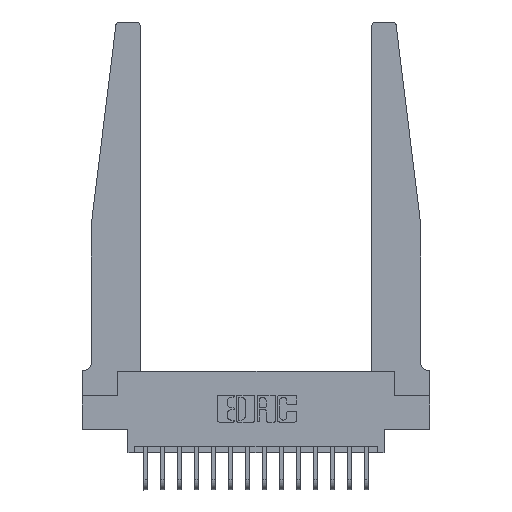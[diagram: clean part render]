
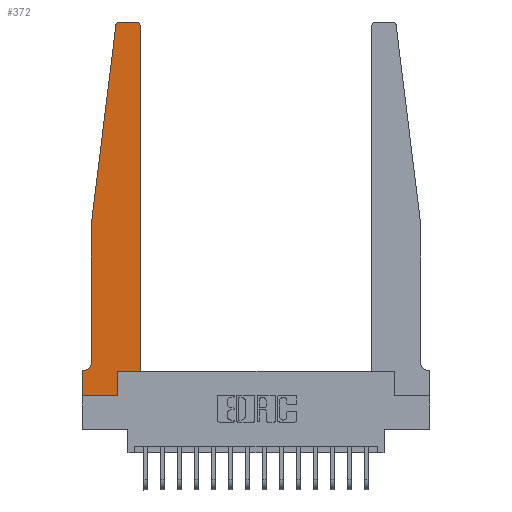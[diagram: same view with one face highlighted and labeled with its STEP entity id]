
A CAD part, top view. The second image highlights one B-rep face of the part: STEP entity #372.
In plain terms, the highlighted planar face has unit normal (0, 0, 1).
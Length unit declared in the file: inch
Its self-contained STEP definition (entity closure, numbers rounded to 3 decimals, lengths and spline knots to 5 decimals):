
#316 = CARTESIAN_POINT ( 'NONE',  ( 0.425, 2.72, 0.37 ) ) ;
#372 = ADVANCED_FACE ( 'NONE', ( #7397 ), #8404, .T. ) ;
#422 = DIRECTION ( 'NONE',  ( 0., -1., 0. ) ) ;
#849 = EDGE_CURVE ( 'NONE', #1952, #6375, #15134, .T. ) ;
#1084 = VERTEX_POINT ( 'NONE', #10043 ) ;
#1203 = DIRECTION ( 'NONE',  ( 1., 0., 0. ) ) ;
#1388 = ORIENTED_EDGE ( 'NONE', *, *, #10476, .T. ) ;
#1481 = DIRECTION ( 'NONE',  ( 1., 0., 0. ) ) ;
#1496 = CARTESIAN_POINT ( 'NONE',  ( 0.065, 1.25, 0.37 ) ) ;
#1817 = LINE ( 'NONE', #8762, #2252 ) ;
#1832 = ORIENTED_EDGE ( 'NONE', *, *, #15131, .T. ) ;
#1952 = VERTEX_POINT ( 'NONE', #4308 ) ;
#2252 = VECTOR ( 'NONE', #422, 39.37008 ) ;
#2431 = VERTEX_POINT ( 'NONE', #12686 ) ;
#2647 = DIRECTION ( 'NONE',  ( 0., 0., 1. ) ) ;
#3090 = EDGE_CURVE ( 'NONE', #2431, #8237, #17460, .T. ) ;
#3104 = CIRCLE ( 'NONE', #5356, 0.03 ) ;
#3363 = CARTESIAN_POINT ( 'NONE',  ( 0.2605, 0., 0.37 ) ) ;
#3645 = VECTOR ( 'NONE', #12883, 39.37008 ) ;
#3650 = DIRECTION ( 'NONE',  ( 0., -1., 0. ) ) ;
#3750 = LINE ( 'NONE', #11215, #17449 ) ;
#3850 = EDGE_CURVE ( 'NONE', #4819, #7649, #10717, .T. ) ;
#3952 = VECTOR ( 'NONE', #7969, 39.37008 ) ;
#3996 = VECTOR ( 'NONE', #4286, 39.37008 ) ;
#4286 = DIRECTION ( 'NONE',  ( -1., 0., 0. ) ) ;
#4308 = CARTESIAN_POINT ( 'NONE',  ( 0.2605, 0.18, 0.37 ) ) ;
#4644 = EDGE_LOOP ( 'NONE', ( #8132, #11613, #5805, #14864, #8345, #15280, #1388, #15687, #1832, #5587, #13024, #16502 ) ) ;
#4819 = VERTEX_POINT ( 'NONE', #11086 ) ;
#5010 = CARTESIAN_POINT ( 'NONE',  ( 0., 0., 0.37 ) ) ;
#5356 = AXIS2_PLACEMENT_3D ( 'NONE', #5907, #15098, #7273 ) ;
#5502 = DIRECTION ( 'NONE',  ( 0., 0., -1. ) ) ;
#5587 = ORIENTED_EDGE ( 'NONE', *, *, #849, .T. ) ;
#5805 = ORIENTED_EDGE ( 'NONE', *, *, #6548, .T. ) ;
#5907 = CARTESIAN_POINT ( 'NONE',  ( 0.395, 2.72, 0.37 ) ) ;
#6087 = EDGE_CURVE ( 'NONE', #7649, #11909, #7371, .T. ) ;
#6375 = VERTEX_POINT ( 'NONE', #15170 ) ;
#6548 = EDGE_CURVE ( 'NONE', #11909, #10144, #7354, .T. ) ;
#6642 = CARTESIAN_POINT ( 'NONE',  ( 0.25, 2.75, 0.37 ) ) ;
#7003 = VERTEX_POINT ( 'NONE', #316 ) ;
#7191 = AXIS2_PLACEMENT_3D ( 'NONE', #13401, #5502, #14726 ) ;
#7273 = DIRECTION ( 'NONE',  ( 1., 0., 0. ) ) ;
#7354 = LINE ( 'NONE', #16759, #3645 ) ;
#7371 = CIRCLE ( 'NONE', #9547, 0.03 ) ;
#7397 = FACE_OUTER_BOUND ( 'NONE', #4644, .T. ) ;
#7649 = VERTEX_POINT ( 'NONE', #15249 ) ;
#7888 = CIRCLE ( 'NONE', #7191, 0.05 ) ;
#7969 = DIRECTION ( 'NONE',  ( -1., 0., 0. ) ) ;
#8132 = ORIENTED_EDGE ( 'NONE', *, *, #3850, .T. ) ;
#8186 = CARTESIAN_POINT ( 'NONE',  ( 0., 0.1875, 0.37 ) ) ;
#8237 = VERTEX_POINT ( 'NONE', #3363 ) ;
#8341 = CARTESIAN_POINT ( 'NONE',  ( 0., 0.1875, 0.37 ) ) ;
#8345 = ORIENTED_EDGE ( 'NONE', *, *, #13932, .T. ) ;
#8404 = PLANE ( 'NONE',  #12423 ) ;
#8734 = EDGE_CURVE ( 'NONE', #10144, #1084, #1817, .T. ) ;
#8762 = CARTESIAN_POINT ( 'NONE',  ( 0.065, 1.25, 0.37 ) ) ;
#9404 = CARTESIAN_POINT ( 'NONE',  ( 0.015, 0.1875, 0.37 ) ) ;
#9446 = VECTOR ( 'NONE', #1203, 39.37008 ) ;
#9547 = AXIS2_PLACEMENT_3D ( 'NONE', #10792, #2647, #12108 ) ;
#9602 = EDGE_CURVE ( 'NONE', #16678, #16761, #14619, .T. ) ;
#9721 = DIRECTION ( 'NONE',  ( 0., 0., 1. ) ) ;
#9798 = CARTESIAN_POINT ( 'NONE',  ( 0.2605, 0.18, 0.37 ) ) ;
#10043 = CARTESIAN_POINT ( 'NONE',  ( 0.065, 0.2375, 0.37 ) ) ;
#10144 = VERTEX_POINT ( 'NONE', #1496 ) ;
#10476 = EDGE_CURVE ( 'NONE', #16761, #2431, #12675, .T. ) ;
#10717 = LINE ( 'NONE', #6642, #3952 ) ;
#10778 = CARTESIAN_POINT ( 'NONE',  ( 0.425, 0.18, 0.37 ) ) ;
#10792 = CARTESIAN_POINT ( 'NONE',  ( 0.27653, 2.72, 0.37 ) ) ;
#11086 = CARTESIAN_POINT ( 'NONE',  ( 0.395, 2.75, 0.37 ) ) ;
#11126 = LINE ( 'NONE', #9798, #14576 ) ;
#11215 = CARTESIAN_POINT ( 'NONE',  ( 0.425, 0.18, 0.37 ) ) ;
#11613 = ORIENTED_EDGE ( 'NONE', *, *, #6087, .T. ) ;
#11909 = VERTEX_POINT ( 'NONE', #14670 ) ;
#12108 = DIRECTION ( 'NONE',  ( 1., 0., 0. ) ) ;
#12423 = AXIS2_PLACEMENT_3D ( 'NONE', #8341, #9721, #1481 ) ;
#12675 = LINE ( 'NONE', #5010, #15738 ) ;
#12686 = CARTESIAN_POINT ( 'NONE',  ( 0., 0., 0.37 ) ) ;
#12883 = DIRECTION ( 'NONE',  ( -0.122, -0.992, 0. ) ) ;
#13024 = ORIENTED_EDGE ( 'NONE', *, *, #16924, .T. ) ;
#13401 = CARTESIAN_POINT ( 'NONE',  ( 0.015, 0.2375, 0.37 ) ) ;
#13596 = CARTESIAN_POINT ( 'NONE',  ( 0.065, 0.1875, 0.37 ) ) ;
#13932 = EDGE_CURVE ( 'NONE', #1084, #16678, #7888, .T. ) ;
#13999 = VECTOR ( 'NONE', #16651, 39.37008 ) ;
#14035 = CARTESIAN_POINT ( 'NONE',  ( 0., 0., 0.37 ) ) ;
#14576 = VECTOR ( 'NONE', #16283, 39.37008 ) ;
#14619 = LINE ( 'NONE', #13596, #3996 ) ;
#14670 = CARTESIAN_POINT ( 'NONE',  ( 0.24675, 2.72367, 0.37 ) ) ;
#14726 = DIRECTION ( 'NONE',  ( -1., 0., 0. ) ) ;
#14864 = ORIENTED_EDGE ( 'NONE', *, *, #8734, .T. ) ;
#15098 = DIRECTION ( 'NONE',  ( 0., 0., 1. ) ) ;
#15131 = EDGE_CURVE ( 'NONE', #8237, #1952, #11126, .T. ) ;
#15134 = LINE ( 'NONE', #10778, #9446 ) ;
#15170 = CARTESIAN_POINT ( 'NONE',  ( 0.425, 0.18, 0.37 ) ) ;
#15249 = CARTESIAN_POINT ( 'NONE',  ( 0.27653, 2.75, 0.37 ) ) ;
#15280 = ORIENTED_EDGE ( 'NONE', *, *, #9602, .T. ) ;
#15687 = ORIENTED_EDGE ( 'NONE', *, *, #3090, .T. ) ;
#15738 = VECTOR ( 'NONE', #3650, 39.37008 ) ;
#16283 = DIRECTION ( 'NONE',  ( 0., 1., 0. ) ) ;
#16299 = EDGE_CURVE ( 'NONE', #7003, #4819, #3104, .T. ) ;
#16494 = DIRECTION ( 'NONE',  ( 0., 1., 0. ) ) ;
#16502 = ORIENTED_EDGE ( 'NONE', *, *, #16299, .T. ) ;
#16651 = DIRECTION ( 'NONE',  ( 1., 0., 0. ) ) ;
#16678 = VERTEX_POINT ( 'NONE', #9404 ) ;
#16759 = CARTESIAN_POINT ( 'NONE',  ( 0.065, 1.25, 0.37 ) ) ;
#16761 = VERTEX_POINT ( 'NONE', #8186 ) ;
#16924 = EDGE_CURVE ( 'NONE', #6375, #7003, #3750, .T. ) ;
#17449 = VECTOR ( 'NONE', #16494, 39.37008 ) ;
#17460 = LINE ( 'NONE', #14035, #13999 ) ;
